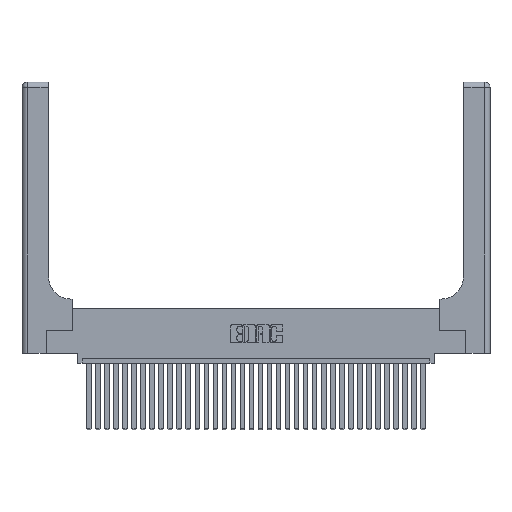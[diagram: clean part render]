
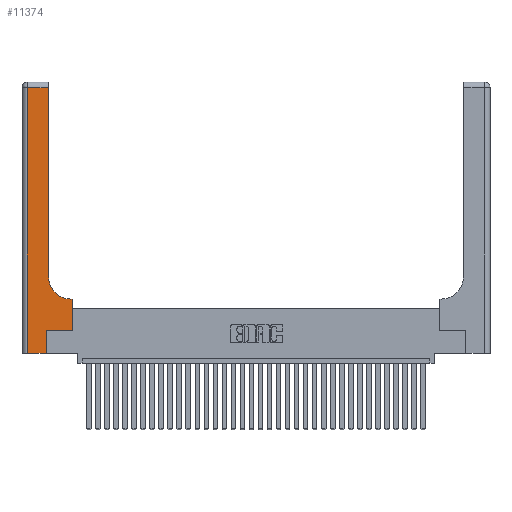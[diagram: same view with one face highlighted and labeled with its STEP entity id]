
A CAD part, top view. The second image highlights one B-rep face of the part: STEP entity #11374.
In plain terms, the highlighted planar face has unit normal (0, 0, 1).
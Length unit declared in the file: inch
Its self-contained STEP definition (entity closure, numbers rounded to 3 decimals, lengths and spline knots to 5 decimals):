
#1721 = LINE ( 'NONE', #18294, #16575 ) ;
#1731 = CARTESIAN_POINT ( 'NONE',  ( 0.2915, 0.6, 0.37 ) ) ;
#2483 = DIRECTION ( 'NONE',  ( 0., 1., 0. ) ) ;
#2745 = VECTOR ( 'NONE', #32536, 39.37008 ) ;
#2750 = CIRCLE ( 'NONE', #12727, 0.25 ) ;
#2827 = CARTESIAN_POINT ( 'NONE',  ( 0.5585, 0.25, 0.37 ) ) ;
#3026 = VERTEX_POINT ( 'NONE', #14066 ) ;
#3029 = LINE ( 'NONE', #3334, #11355 ) ;
#3334 = CARTESIAN_POINT ( 'NONE',  ( 0.2915, 3., 0.37 ) ) ;
#4372 = EDGE_CURVE ( 'NONE', #14198, #3026, #24115, .T. ) ;
#4622 = CARTESIAN_POINT ( 'NONE',  ( 0.269, 0., 0.37 ) ) ;
#4927 = PLANE ( 'NONE',  #29976 ) ;
#5460 = EDGE_CURVE ( 'NONE', #27870, #14198, #1721, .T. ) ;
#5483 = CARTESIAN_POINT ( 'NONE',  ( 0.5585, 0.25, 0.37 ) ) ;
#5516 = VERTEX_POINT ( 'NONE', #18840 ) ;
#5900 = CARTESIAN_POINT ( 'NONE',  ( 0.2915, 2.94, 0.37 ) ) ;
#6014 = EDGE_CURVE ( 'NONE', #3026, #14471, #12859, .T. ) ;
#6246 = ORIENTED_EDGE ( 'NONE', *, *, #27351, .T. ) ;
#6771 = VECTOR ( 'NONE', #2483, 39.37008 ) ;
#6904 = VERTEX_POINT ( 'NONE', #16834 ) ;
#7409 = CARTESIAN_POINT ( 'NONE',  ( 0.06, 0., 0.37 ) ) ;
#7641 = LINE ( 'NONE', #31006, #20849 ) ;
#8690 = VECTOR ( 'NONE', #28620, 39.37008 ) ;
#9928 = EDGE_LOOP ( 'NONE', ( #6246, #17097, #14466, #14437, #17343, #31130, #22009, #17300, #22576 ) ) ;
#10284 = CARTESIAN_POINT ( 'NONE',  ( 0., 2.94, 0.37 ) ) ;
#11355 = VECTOR ( 'NONE', #13998, 39.37008 ) ;
#11374 = ADVANCED_FACE ( 'NONE', ( #32791 ), #4927, .F. ) ;
#12350 = CARTESIAN_POINT ( 'NONE',  ( 0.269, 0.25, 0.37 ) ) ;
#12600 = DIRECTION ( 'NONE',  ( 0., 1., 0. ) ) ;
#12670 = EDGE_CURVE ( 'NONE', #5516, #27870, #25231, .T. ) ;
#12727 = AXIS2_PLACEMENT_3D ( 'NONE', #17455, #17111, #25305 ) ;
#12859 = LINE ( 'NONE', #1731, #8690 ) ;
#13942 = CARTESIAN_POINT ( 'NONE',  ( 0.06, 3., 0.37 ) ) ;
#13998 = DIRECTION ( 'NONE',  ( 0., 1., 0. ) ) ;
#14066 = CARTESIAN_POINT ( 'NONE',  ( 0.5585, 0.6, 0.37 ) ) ;
#14198 = VERTEX_POINT ( 'NONE', #2827 ) ;
#14437 = ORIENTED_EDGE ( 'NONE', *, *, #27677, .T. ) ;
#14466 = ORIENTED_EDGE ( 'NONE', *, *, #32172, .T. ) ;
#14471 = VERTEX_POINT ( 'NONE', #23306 ) ;
#15680 = DIRECTION ( 'NONE',  ( 0., 0., -1. ) ) ;
#16029 = VECTOR ( 'NONE', #25845, 39.37008 ) ;
#16575 = VECTOR ( 'NONE', #17961, 39.37008 ) ;
#16834 = CARTESIAN_POINT ( 'NONE',  ( 0.2915, 0.85, 0.37 ) ) ;
#17097 = ORIENTED_EDGE ( 'NONE', *, *, #18850, .T. ) ;
#17111 = DIRECTION ( 'NONE',  ( 0., 0., -1. ) ) ;
#17300 = ORIENTED_EDGE ( 'NONE', *, *, #6014, .T. ) ;
#17343 = ORIENTED_EDGE ( 'NONE', *, *, #12670, .T. ) ;
#17455 = CARTESIAN_POINT ( 'NONE',  ( 0.5415, 0.85, 0.37 ) ) ;
#17961 = DIRECTION ( 'NONE',  ( 1., 0., 0. ) ) ;
#18294 = CARTESIAN_POINT ( 'NONE',  ( 0.269, 0.25, 0.37 ) ) ;
#18833 = VERTEX_POINT ( 'NONE', #28594 ) ;
#18840 = CARTESIAN_POINT ( 'NONE',  ( 0.269, 0., 0.37 ) ) ;
#18850 = EDGE_CURVE ( 'NONE', #30445, #18833, #23075, .T. ) ;
#19894 = EDGE_CURVE ( 'NONE', #14471, #6904, #2750, .T. ) ;
#20849 = VECTOR ( 'NONE', #31107, 39.37008 ) ;
#22009 = ORIENTED_EDGE ( 'NONE', *, *, #4372, .T. ) ;
#22576 = ORIENTED_EDGE ( 'NONE', *, *, #19894, .T. ) ;
#23075 = LINE ( 'NONE', #10284, #16029 ) ;
#23192 = DIRECTION ( 'NONE',  ( -1., 0., 0. ) ) ;
#23306 = CARTESIAN_POINT ( 'NONE',  ( 0.5415, 0.6, 0.37 ) ) ;
#24115 = LINE ( 'NONE', #5483, #6771 ) ;
#25231 = LINE ( 'NONE', #4622, #31449 ) ;
#25305 = DIRECTION ( 'NONE',  ( 1., 0., 0. ) ) ;
#25845 = DIRECTION ( 'NONE',  ( -1., 0., 0. ) ) ;
#26317 = LINE ( 'NONE', #13942, #2745 ) ;
#27351 = EDGE_CURVE ( 'NONE', #6904, #30445, #3029, .T. ) ;
#27677 = EDGE_CURVE ( 'NONE', #29652, #5516, #7641, .T. ) ;
#27870 = VERTEX_POINT ( 'NONE', #12350 ) ;
#28594 = CARTESIAN_POINT ( 'NONE',  ( 0.06, 2.94, 0.37 ) ) ;
#28620 = DIRECTION ( 'NONE',  ( -1., 0., 0. ) ) ;
#28799 = CARTESIAN_POINT ( 'NONE',  ( 0., 3., 0.37 ) ) ;
#29652 = VERTEX_POINT ( 'NONE', #7409 ) ;
#29976 = AXIS2_PLACEMENT_3D ( 'NONE', #28799, #15680, #23192 ) ;
#30445 = VERTEX_POINT ( 'NONE', #5900 ) ;
#31006 = CARTESIAN_POINT ( 'NONE',  ( 0., 0., 0.37 ) ) ;
#31107 = DIRECTION ( 'NONE',  ( 1., 0., 0. ) ) ;
#31130 = ORIENTED_EDGE ( 'NONE', *, *, #5460, .T. ) ;
#31449 = VECTOR ( 'NONE', #12600, 39.37008 ) ;
#32172 = EDGE_CURVE ( 'NONE', #18833, #29652, #26317, .T. ) ;
#32536 = DIRECTION ( 'NONE',  ( 0., -1., 0. ) ) ;
#32791 = FACE_OUTER_BOUND ( 'NONE', #9928, .T. ) ;
